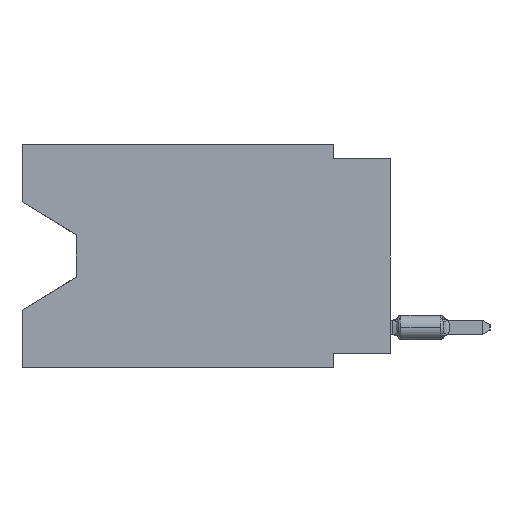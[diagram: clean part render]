
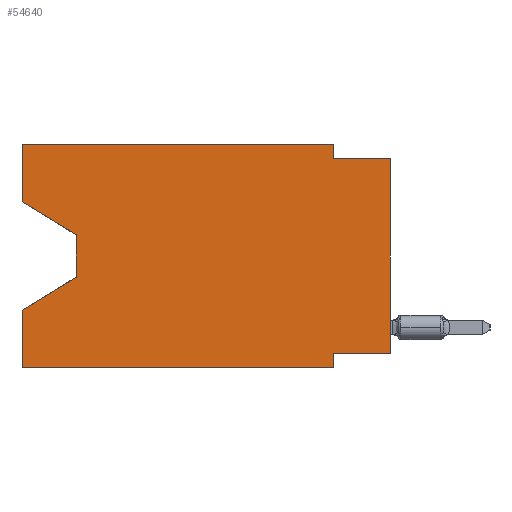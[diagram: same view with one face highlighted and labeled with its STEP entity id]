
A CAD part, left-side view. The second image highlights one B-rep face of the part: STEP entity #54640.
In plain terms, the highlighted planar face has unit normal (-1, 0, 0).
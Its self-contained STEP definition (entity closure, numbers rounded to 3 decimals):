
#348 = DIRECTION ( 'NONE',  ( 0., -1., 0. ) ) ;
#1336 = DIRECTION ( 'NONE',  ( 0., 0., -1. ) ) ;
#1731 = VECTOR ( 'NONE', #31453, 1000. ) ;
#2740 = VECTOR ( 'NONE', #348, 1000. ) ;
#4434 = DIRECTION ( 'NONE',  ( 0., 0., 1. ) ) ;
#4596 = CARTESIAN_POINT ( 'NONE',  ( 0., 2.54, 0. ) ) ;
#4805 = LINE ( 'NONE', #10541, #64389 ) ;
#4950 = VERTEX_POINT ( 'NONE', #5458 ) ;
#5458 = CARTESIAN_POINT ( 'NONE',  ( 0., 0., -0.635 ) ) ;
#6955 = EDGE_CURVE ( 'NONE', #34442, #36792, #55920, .T. ) ;
#8545 = VERTEX_POINT ( 'NONE', #23783 ) ;
#8770 = VERTEX_POINT ( 'NONE', #73888 ) ;
#9402 = VECTOR ( 'NONE', #38917, 1000. ) ;
#9652 = EDGE_CURVE ( 'NONE', #11926, #4950, #33828, .T. ) ;
#9702 = FACE_OUTER_BOUND ( 'NONE', #14822, .T. ) ;
#10541 = CARTESIAN_POINT ( 'NONE',  ( 0., 16.383, 0. ) ) ;
#11309 = DIRECTION ( 'NONE',  ( 0., -0.855, -0.519 ) ) ;
#11926 = VERTEX_POINT ( 'NONE', #29185 ) ;
#12132 = ORIENTED_EDGE ( 'NONE', *, *, #21620, .T. ) ;
#13353 = CARTESIAN_POINT ( 'NONE',  ( 0., 2.54, -9.906 ) ) ;
#13421 = DIRECTION ( 'NONE',  ( 0., 0., -1. ) ) ;
#13643 = VECTOR ( 'NONE', #15645, 1000. ) ;
#14194 = LINE ( 'NONE', #72844, #1731 ) ;
#14535 = DIRECTION ( 'NONE',  ( 0., 0., 1. ) ) ;
#14822 = EDGE_LOOP ( 'NONE', ( #43624, #12132, #40819, #27237, #74707, #27111, #56601, #46763, #68716, #58939, #31209, #51472 ) ) ;
#15085 = LINE ( 'NONE', #46784, #15280 ) ;
#15280 = VECTOR ( 'NONE', #67619, 1000. ) ;
#15645 = DIRECTION ( 'NONE',  ( 0., -1., 0. ) ) ;
#16860 = CARTESIAN_POINT ( 'NONE',  ( 0., 2.54, -9.271 ) ) ;
#21562 = PLANE ( 'NONE',  #39206 ) ;
#21620 = EDGE_CURVE ( 'NONE', #60907, #8545, #71685, .T. ) ;
#23783 = CARTESIAN_POINT ( 'NONE',  ( 0., 13.97, -5.893 ) ) ;
#26183 = VECTOR ( 'NONE', #34101, 1000. ) ;
#27111 = ORIENTED_EDGE ( 'NONE', *, *, #70545, .F. ) ;
#27237 = ORIENTED_EDGE ( 'NONE', *, *, #75836, .F. ) ;
#28127 = VECTOR ( 'NONE', #11309, 1000. ) ;
#29185 = CARTESIAN_POINT ( 'NONE',  ( 0., 0., -9.271 ) ) ;
#29775 = CARTESIAN_POINT ( 'NONE',  ( 0., 16.383, 0. ) ) ;
#30753 = VERTEX_POINT ( 'NONE', #29775 ) ;
#31209 = ORIENTED_EDGE ( 'NONE', *, *, #45301, .F. ) ;
#31453 = DIRECTION ( 'NONE',  ( 0., 0.855, -0.519 ) ) ;
#33828 = LINE ( 'NONE', #57198, #51918 ) ;
#34101 = DIRECTION ( 'NONE',  ( 0., 0., -1. ) ) ;
#34442 = VERTEX_POINT ( 'NONE', #43652 ) ;
#35762 = CARTESIAN_POINT ( 'NONE',  ( 0., 16.383, 0. ) ) ;
#35938 = CARTESIAN_POINT ( 'NONE',  ( 0., 16.383, -7.36 ) ) ;
#36792 = VERTEX_POINT ( 'NONE', #13353 ) ;
#36947 = VECTOR ( 'NONE', #14535, 1000. ) ;
#38917 = DIRECTION ( 'NONE',  ( 0., -1., 0. ) ) ;
#39206 = AXIS2_PLACEMENT_3D ( 'NONE', #51094, #45718, #69096 ) ;
#40819 = ORIENTED_EDGE ( 'NONE', *, *, #47069, .T. ) ;
#40901 = VERTEX_POINT ( 'NONE', #46953 ) ;
#41345 = CARTESIAN_POINT ( 'NONE',  ( 0., 2.54, -0.635 ) ) ;
#42488 = CARTESIAN_POINT ( 'NONE',  ( 0., 16.383, 0. ) ) ;
#42560 = CARTESIAN_POINT ( 'NONE',  ( 0., 13.97, -4.013 ) ) ;
#42919 = LINE ( 'NONE', #35762, #36947 ) ;
#43624 = ORIENTED_EDGE ( 'NONE', *, *, #53774, .T. ) ;
#43652 = CARTESIAN_POINT ( 'NONE',  ( 0., 16.383, -9.906 ) ) ;
#44997 = VECTOR ( 'NONE', #1336, 1000. ) ;
#45029 = LINE ( 'NONE', #68408, #9402 ) ;
#45301 = EDGE_CURVE ( 'NONE', #30753, #40901, #59363, .T. ) ;
#45718 = DIRECTION ( 'NONE',  ( 1., 0., 0. ) ) ;
#46763 = ORIENTED_EDGE ( 'NONE', *, *, #9652, .T. ) ;
#46784 = CARTESIAN_POINT ( 'NONE',  ( 0., 0., -9.271 ) ) ;
#46892 = CARTESIAN_POINT ( 'NONE',  ( 0., 13.97, -4.013 ) ) ;
#46953 = CARTESIAN_POINT ( 'NONE',  ( 0., 2.54, 0. ) ) ;
#47069 = EDGE_CURVE ( 'NONE', #8545, #58908, #14194, .T. ) ;
#47258 = EDGE_CURVE ( 'NONE', #40901, #61676, #63981, .T. ) ;
#49319 = EDGE_CURVE ( 'NONE', #8770, #30753, #4805, .T. ) ;
#50284 = EDGE_CURVE ( 'NONE', #61676, #4950, #45029, .T. ) ;
#51094 = CARTESIAN_POINT ( 'NONE',  ( 0., 16.383, 0. ) ) ;
#51442 = DIRECTION ( 'NONE',  ( 0., 0., 1. ) ) ;
#51472 = ORIENTED_EDGE ( 'NONE', *, *, #49319, .F. ) ;
#51918 = VECTOR ( 'NONE', #51442, 1000. ) ;
#52712 = LINE ( 'NONE', #75331, #28127 ) ;
#53774 = EDGE_CURVE ( 'NONE', #8770, #60907, #52712, .T. ) ;
#54640 = ADVANCED_FACE ( 'NONE', ( #9702 ), #21562, .F. ) ;
#55920 = LINE ( 'NONE', #67803, #13643 ) ;
#56601 = ORIENTED_EDGE ( 'NONE', *, *, #58341, .F. ) ;
#57198 = CARTESIAN_POINT ( 'NONE',  ( 0., 0., 0. ) ) ;
#58334 = VERTEX_POINT ( 'NONE', #16860 ) ;
#58341 = EDGE_CURVE ( 'NONE', #11926, #58334, #15085, .T. ) ;
#58908 = VERTEX_POINT ( 'NONE', #35938 ) ;
#58939 = ORIENTED_EDGE ( 'NONE', *, *, #47258, .F. ) ;
#59363 = LINE ( 'NONE', #42488, #2740 ) ;
#59609 = LINE ( 'NONE', #60742, #44997 ) ;
#60742 = CARTESIAN_POINT ( 'NONE',  ( 0., 2.54, -9.906 ) ) ;
#60907 = VERTEX_POINT ( 'NONE', #46892 ) ;
#61676 = VERTEX_POINT ( 'NONE', #41345 ) ;
#63981 = LINE ( 'NONE', #4596, #26183 ) ;
#64331 = VECTOR ( 'NONE', #13421, 1000. ) ;
#64389 = VECTOR ( 'NONE', #4434, 1000. ) ;
#67619 = DIRECTION ( 'NONE',  ( 0., 1., 0. ) ) ;
#67803 = CARTESIAN_POINT ( 'NONE',  ( 0., 16.383, -9.906 ) ) ;
#68408 = CARTESIAN_POINT ( 'NONE',  ( 0., 0., -0.635 ) ) ;
#68716 = ORIENTED_EDGE ( 'NONE', *, *, #50284, .F. ) ;
#69096 = DIRECTION ( 'NONE',  ( 0., 0., -1. ) ) ;
#70545 = EDGE_CURVE ( 'NONE', #58334, #36792, #59609, .T. ) ;
#71685 = LINE ( 'NONE', #42560, #64331 ) ;
#72844 = CARTESIAN_POINT ( 'NONE',  ( 0., 13.97, -5.893 ) ) ;
#73888 = CARTESIAN_POINT ( 'NONE',  ( 0., 16.383, -2.546 ) ) ;
#74707 = ORIENTED_EDGE ( 'NONE', *, *, #6955, .T. ) ;
#75331 = CARTESIAN_POINT ( 'NONE',  ( 0., 16.383, -2.546 ) ) ;
#75836 = EDGE_CURVE ( 'NONE', #34442, #58908, #42919, .T. ) ;
